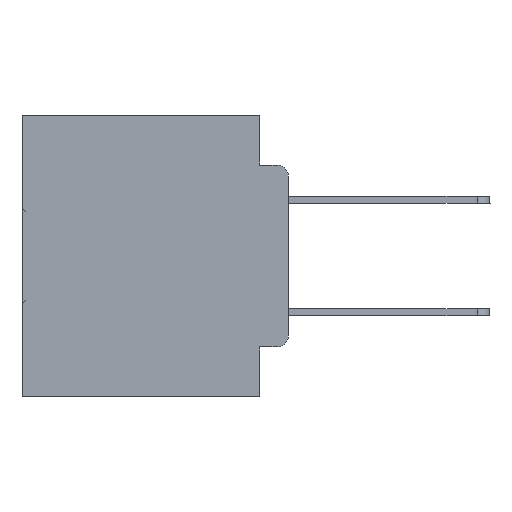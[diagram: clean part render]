
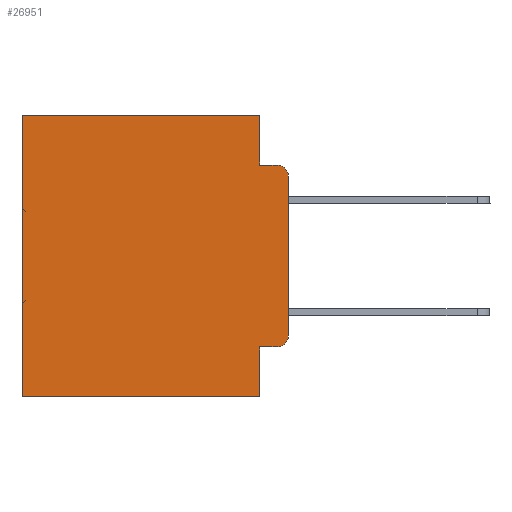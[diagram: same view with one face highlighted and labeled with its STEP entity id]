
A CAD part, left-side view. The second image highlights one B-rep face of the part: STEP entity #26951.
In plain terms, the highlighted planar face has unit normal (-1, 0, 0).
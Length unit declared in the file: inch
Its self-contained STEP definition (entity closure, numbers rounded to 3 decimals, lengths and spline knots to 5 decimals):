
#376 = VERTEX_POINT ( 'NONE', #23762 ) ;
#929 = CARTESIAN_POINT ( 'NONE',  ( 0.298, 0.051, -0.0885 ) ) ;
#1178 = VECTOR ( 'NONE', #25832, 39.37008 ) ;
#2679 = VECTOR ( 'NONE', #32584, 39.37008 ) ;
#2823 = CARTESIAN_POINT ( 'NONE',  ( 0.298, 0.051, -0.4115 ) ) ;
#2950 = VECTOR ( 'NONE', #10990, 39.37008 ) ;
#3091 = CARTESIAN_POINT ( 'NONE',  ( 0.298, 0.473, 0. ) ) ;
#3544 = EDGE_CURVE ( 'NONE', #18085, #9387, #8738, .T. ) ;
#4108 = CARTESIAN_POINT ( 'NONE',  ( 0.298, 0., -0.3915 ) ) ;
#4516 = CARTESIAN_POINT ( 'NONE',  ( 0.298, 0.02, -0.1085 ) ) ;
#4623 = VECTOR ( 'NONE', #26046, 39.37008 ) ;
#4658 = VECTOR ( 'NONE', #7849, 39.37008 ) ;
#7038 = EDGE_CURVE ( 'NONE', #32162, #376, #34047, .T. ) ;
#7649 = EDGE_CURVE ( 'NONE', #29252, #33546, #34617, .T. ) ;
#7849 = DIRECTION ( 'NONE',  ( 0., 1., 0. ) ) ;
#8396 = ORIENTED_EDGE ( 'NONE', *, *, #29473, .T. ) ;
#8738 = LINE ( 'NONE', #23468, #1178 ) ;
#9053 = ORIENTED_EDGE ( 'NONE', *, *, #3544, .T. ) ;
#9387 = VERTEX_POINT ( 'NONE', #21355 ) ;
#9560 = ORIENTED_EDGE ( 'NONE', *, *, #11038, .F. ) ;
#9731 = VECTOR ( 'NONE', #21465, 39.37008 ) ;
#9830 = EDGE_CURVE ( 'NONE', #32162, #29252, #10087, .T. ) ;
#10087 = LINE ( 'NONE', #2823, #2950 ) ;
#10361 = VECTOR ( 'NONE', #13332, 39.37008 ) ;
#10628 = CARTESIAN_POINT ( 'NONE',  ( 0.298, 0.051, 0. ) ) ;
#10674 = CARTESIAN_POINT ( 'NONE',  ( 0.298, 0.051, 0. ) ) ;
#10960 = DIRECTION ( 'NONE',  ( 0., 0., -1. ) ) ;
#10990 = DIRECTION ( 'NONE',  ( 0., -1., 0. ) ) ;
#11038 = EDGE_CURVE ( 'NONE', #18085, #24460, #27529, .T. ) ;
#11344 = ORIENTED_EDGE ( 'NONE', *, *, #34282, .F. ) ;
#11591 = CARTESIAN_POINT ( 'NONE',  ( 0.298, 0., 0. ) ) ;
#12783 = VERTEX_POINT ( 'NONE', #34446 ) ;
#13317 = CARTESIAN_POINT ( 'NONE',  ( 0.298, 0.02, -0.4115 ) ) ;
#13332 = DIRECTION ( 'NONE',  ( 0., 0., -1. ) ) ;
#14432 = DIRECTION ( 'NONE',  ( 1., 0., 0. ) ) ;
#15917 = EDGE_CURVE ( 'NONE', #34001, #33546, #17503, .T. ) ;
#17503 = LINE ( 'NONE', #23028, #10361 ) ;
#17902 = EDGE_CURVE ( 'NONE', #9387, #12783, #33724, .T. ) ;
#18085 = VERTEX_POINT ( 'NONE', #30441 ) ;
#19146 = AXIS2_PLACEMENT_3D ( 'NONE', #11591, #14432, #30300 ) ;
#19901 = ORIENTED_EDGE ( 'NONE', *, *, #7038, .F. ) ;
#20077 = DIRECTION ( 'NONE',  ( -1., 0., 0. ) ) ;
#20440 = ORIENTED_EDGE ( 'NONE', *, *, #9830, .T. ) ;
#20878 = ORIENTED_EDGE ( 'NONE', *, *, #15917, .F. ) ;
#21035 = CARTESIAN_POINT ( 'NONE',  ( 0.298, 0.051, -0.4115 ) ) ;
#21355 = CARTESIAN_POINT ( 'NONE',  ( 0.298, 0.473, 0. ) ) ;
#21465 = DIRECTION ( 'NONE',  ( 0., 0., -1. ) ) ;
#21812 = FACE_OUTER_BOUND ( 'NONE', #33349, .T. ) ;
#22219 = LINE ( 'NONE', #26399, #4623 ) ;
#23028 = CARTESIAN_POINT ( 'NONE',  ( 0.298, 0., 0. ) ) ;
#23244 = DIRECTION ( 'NONE',  ( 0., 0., -1. ) ) ;
#23306 = CIRCLE ( 'NONE', #27959, 0.02 ) ;
#23355 = VECTOR ( 'NONE', #10960, 39.37008 ) ;
#23468 = CARTESIAN_POINT ( 'NONE',  ( 0.298, 0., 0. ) ) ;
#23762 = CARTESIAN_POINT ( 'NONE',  ( 0.298, 0.051, -0.5 ) ) ;
#24460 = VERTEX_POINT ( 'NONE', #929 ) ;
#24488 = AXIS2_PLACEMENT_3D ( 'NONE', #25672, #20077, #30924 ) ;
#25672 = CARTESIAN_POINT ( 'NONE',  ( 0.298, 0.02, -0.3915 ) ) ;
#25832 = DIRECTION ( 'NONE',  ( 0., 1., 0. ) ) ;
#26046 = DIRECTION ( 'NONE',  ( 0., -1., 0. ) ) ;
#26109 = VERTEX_POINT ( 'NONE', #32419 ) ;
#26113 = EDGE_CURVE ( 'NONE', #376, #12783, #34452, .T. ) ;
#26399 = CARTESIAN_POINT ( 'NONE',  ( 0.298, 0.051, -0.0885 ) ) ;
#26777 = CARTESIAN_POINT ( 'NONE',  ( 0.298, 0., -0.5 ) ) ;
#26951 = ADVANCED_FACE ( 'NONE', ( #21812 ), #30766, .F. ) ;
#27529 = LINE ( 'NONE', #10628, #23355 ) ;
#27670 = DIRECTION ( 'NONE',  ( -1., 0., 0. ) ) ;
#27959 = AXIS2_PLACEMENT_3D ( 'NONE', #4516, #27670, #23244 ) ;
#29044 = ORIENTED_EDGE ( 'NONE', *, *, #17902, .T. ) ;
#29252 = VERTEX_POINT ( 'NONE', #13317 ) ;
#29473 = EDGE_CURVE ( 'NONE', #34001, #26109, #23306, .T. ) ;
#30300 = DIRECTION ( 'NONE',  ( 0., 0., -1. ) ) ;
#30441 = CARTESIAN_POINT ( 'NONE',  ( 0.298, 0.051, 0. ) ) ;
#30766 = PLANE ( 'NONE',  #19146 ) ;
#30924 = DIRECTION ( 'NONE',  ( 0., 0., -1. ) ) ;
#32162 = VERTEX_POINT ( 'NONE', #21035 ) ;
#32419 = CARTESIAN_POINT ( 'NONE',  ( 0.298, 0.02, -0.0885 ) ) ;
#32584 = DIRECTION ( 'NONE',  ( 0., 0., -1. ) ) ;
#32615 = ORIENTED_EDGE ( 'NONE', *, *, #26113, .F. ) ;
#33000 = CARTESIAN_POINT ( 'NONE',  ( 0.298, 0., -0.1085 ) ) ;
#33349 = EDGE_LOOP ( 'NONE', ( #20878, #8396, #11344, #9560, #9053, #29044, #32615, #19901, #20440, #34643 ) ) ;
#33546 = VERTEX_POINT ( 'NONE', #4108 ) ;
#33724 = LINE ( 'NONE', #3091, #2679 ) ;
#34001 = VERTEX_POINT ( 'NONE', #33000 ) ;
#34047 = LINE ( 'NONE', #10674, #9731 ) ;
#34282 = EDGE_CURVE ( 'NONE', #24460, #26109, #22219, .T. ) ;
#34446 = CARTESIAN_POINT ( 'NONE',  ( 0.298, 0.473, -0.5 ) ) ;
#34452 = LINE ( 'NONE', #26777, #4658 ) ;
#34617 = CIRCLE ( 'NONE', #24488, 0.02 ) ;
#34643 = ORIENTED_EDGE ( 'NONE', *, *, #7649, .T. ) ;
